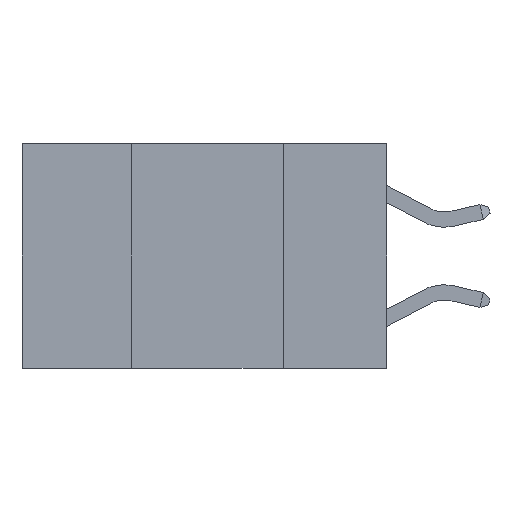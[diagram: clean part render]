
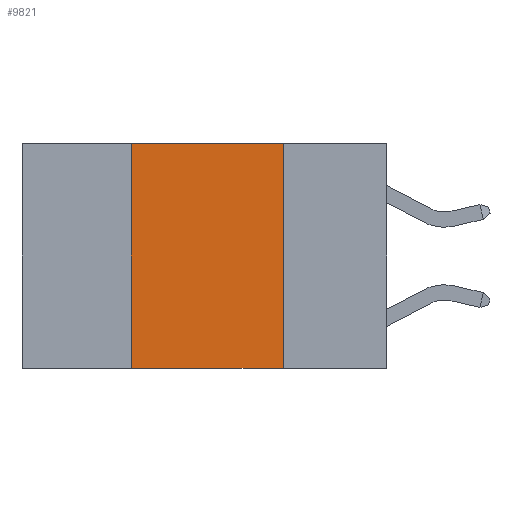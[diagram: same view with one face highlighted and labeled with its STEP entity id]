
A CAD part, left-side view. The second image highlights one B-rep face of the part: STEP entity #9821.
In plain terms, the highlighted planar face has unit normal (-1, 0, 0).
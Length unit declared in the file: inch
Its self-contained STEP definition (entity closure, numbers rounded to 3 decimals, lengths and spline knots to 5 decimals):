
#786 = EDGE_CURVE ( 'NONE', #9200, #1596, #6343, .T. ) ;
#1362 = CARTESIAN_POINT ( 'NONE',  ( 0., 0.42, 0. ) ) ;
#1596 = VERTEX_POINT ( 'NONE', #3480 ) ;
#1685 = DIRECTION ( 'NONE',  ( 0., 0., -1. ) ) ;
#2164 = FACE_OUTER_BOUND ( 'NONE', #13440, .T. ) ;
#2798 = CARTESIAN_POINT ( 'NONE',  ( 0., 0.17, 0. ) ) ;
#2942 = VECTOR ( 'NONE', #11498, 39.37008 ) ;
#3015 = EDGE_CURVE ( 'NONE', #9200, #15152, #8880, .T. ) ;
#3187 = DIRECTION ( 'NONE',  ( 0., -1., 0. ) ) ;
#3480 = CARTESIAN_POINT ( 'NONE',  ( 0., 0.17, -0.37 ) ) ;
#3726 = VERTEX_POINT ( 'NONE', #2798 ) ;
#5329 = EDGE_CURVE ( 'NONE', #15152, #3726, #6845, .T. ) ;
#5390 = CARTESIAN_POINT ( 'NONE',  ( 0., 0.17, 0. ) ) ;
#5832 = LINE ( 'NONE', #5390, #12935 ) ;
#6093 = EDGE_CURVE ( 'NONE', #3726, #1596, #5832, .T. ) ;
#6343 = LINE ( 'NONE', #6948, #16138 ) ;
#6845 = LINE ( 'NONE', #13663, #13164 ) ;
#6948 = CARTESIAN_POINT ( 'NONE',  ( 0., 0.6, -0.37 ) ) ;
#7989 = ORIENTED_EDGE ( 'NONE', *, *, #5329, .F. ) ;
#7992 = CARTESIAN_POINT ( 'NONE',  ( 0., 0.6, 0. ) ) ;
#8880 = LINE ( 'NONE', #1362, #2942 ) ;
#9200 = VERTEX_POINT ( 'NONE', #14307 ) ;
#9300 = DIRECTION ( 'NONE',  ( 1., 0., 0. ) ) ;
#9821 = ADVANCED_FACE ( 'NONE', ( #2164 ), #15646, .F. ) ;
#11129 = CARTESIAN_POINT ( 'NONE',  ( 0., 0.42, 0. ) ) ;
#11351 = ORIENTED_EDGE ( 'NONE', *, *, #3015, .F. ) ;
#11498 = DIRECTION ( 'NONE',  ( 0., 0., 1. ) ) ;
#12630 = AXIS2_PLACEMENT_3D ( 'NONE', #7992, #9300, #1685 ) ;
#12935 = VECTOR ( 'NONE', #14275, 39.37008 ) ;
#13164 = VECTOR ( 'NONE', #14975, 39.37008 ) ;
#13440 = EDGE_LOOP ( 'NONE', ( #14379, #7989, #11351, #14782 ) ) ;
#13663 = CARTESIAN_POINT ( 'NONE',  ( 0., 0.6, 0. ) ) ;
#14275 = DIRECTION ( 'NONE',  ( 0., 0., -1. ) ) ;
#14307 = CARTESIAN_POINT ( 'NONE',  ( 0., 0.42, -0.37 ) ) ;
#14379 = ORIENTED_EDGE ( 'NONE', *, *, #6093, .F. ) ;
#14782 = ORIENTED_EDGE ( 'NONE', *, *, #786, .T. ) ;
#14975 = DIRECTION ( 'NONE',  ( 0., -1., 0. ) ) ;
#15152 = VERTEX_POINT ( 'NONE', #11129 ) ;
#15646 = PLANE ( 'NONE',  #12630 ) ;
#16138 = VECTOR ( 'NONE', #3187, 39.37008 ) ;
